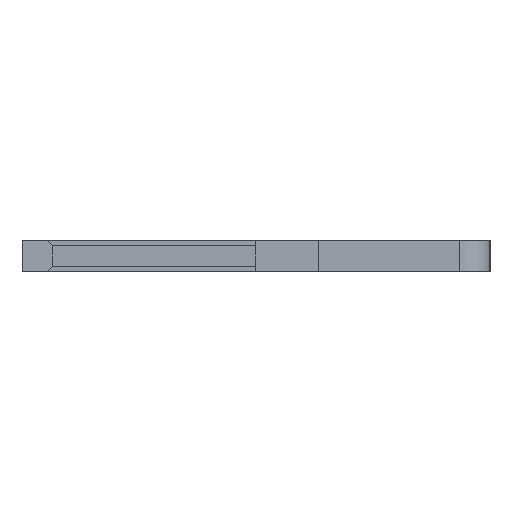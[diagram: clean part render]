
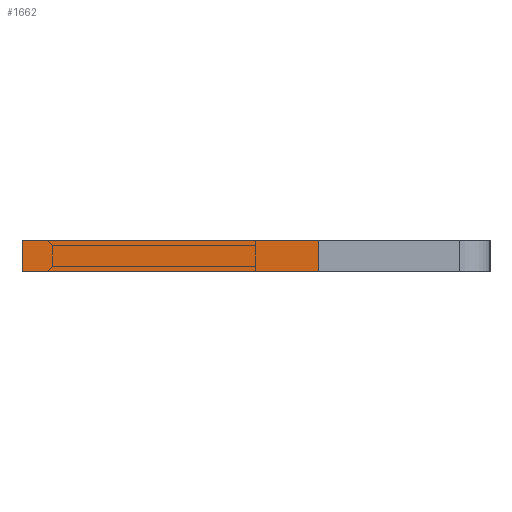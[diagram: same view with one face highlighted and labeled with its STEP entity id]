
A CAD part, left-side view. The second image highlights one B-rep face of the part: STEP entity #1662.
In plain terms, the highlighted face is planar.
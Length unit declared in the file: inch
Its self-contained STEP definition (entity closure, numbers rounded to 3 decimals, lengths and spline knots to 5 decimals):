
#30 = EDGE_CURVE ( 'NONE', #1767, #57, #1010, .T. ) ;
#57 = VERTEX_POINT ( 'NONE', #2047 ) ;
#97 = VECTOR ( 'NONE', #1008, 39.37008 ) ;
#149 = DIRECTION ( 'NONE',  ( 0., 0., 1. ) ) ;
#417 = DIRECTION ( 'NONE',  ( 0., 1., 0. ) ) ;
#457 = CARTESIAN_POINT ( 'NONE',  ( 0.01, 0.15, -0.04 ) ) ;
#492 = FACE_OUTER_BOUND ( 'NONE', #2109, .T. ) ;
#567 = LINE ( 'NONE', #1866, #97 ) ;
#683 = ORIENTED_EDGE ( 'NONE', *, *, #30, .F. ) ;
#798 = LINE ( 'NONE', #1511, #913 ) ;
#806 = EDGE_CURVE ( 'NONE', #2114, #57, #1166, .T. ) ;
#818 = DIRECTION ( 'NONE',  ( 1., 0., 0. ) ) ;
#913 = VECTOR ( 'NONE', #1022, 39.37008 ) ;
#996 = VERTEX_POINT ( 'NONE', #1268 ) ;
#1008 = DIRECTION ( 'NONE',  ( -1., 0., 0. ) ) ;
#1010 = LINE ( 'NONE', #1528, #1907 ) ;
#1022 = DIRECTION ( 'NONE',  ( 0., 1., 0. ) ) ;
#1028 = CARTESIAN_POINT ( 'NONE',  ( -0.01, -0.04, -0.04 ) ) ;
#1048 = AXIS2_PLACEMENT_3D ( 'NONE', #457, #149, #818 ) ;
#1166 = LINE ( 'NONE', #1278, #2105 ) ;
#1176 = ORIENTED_EDGE ( 'NONE', *, *, #1977, .F. ) ;
#1268 = CARTESIAN_POINT ( 'NONE',  ( 0.01, -0.04, -0.04 ) ) ;
#1278 = CARTESIAN_POINT ( 'NONE',  ( -0.01, 0.15, -0.04 ) ) ;
#1342 = PLANE ( 'NONE',  #1048 ) ;
#1493 = CARTESIAN_POINT ( 'NONE',  ( 0.01, 0.15, -0.04 ) ) ;
#1511 = CARTESIAN_POINT ( 'NONE',  ( 0.01, 0.15, -0.04 ) ) ;
#1528 = CARTESIAN_POINT ( 'NONE',  ( 0.01, 0.15, -0.04 ) ) ;
#1531 = ORIENTED_EDGE ( 'NONE', *, *, #1799, .T. ) ;
#1547 = DIRECTION ( 'NONE',  ( -1., 0., 0. ) ) ;
#1662 = ADVANCED_FACE ( 'NONE', ( #492 ), #1342, .F. ) ;
#1767 = VERTEX_POINT ( 'NONE', #1493 ) ;
#1799 = EDGE_CURVE ( 'NONE', #996, #2114, #567, .T. ) ;
#1805 = ORIENTED_EDGE ( 'NONE', *, *, #806, .T. ) ;
#1866 = CARTESIAN_POINT ( 'NONE',  ( 0.01, -0.04, -0.04 ) ) ;
#1907 = VECTOR ( 'NONE', #1547, 39.37008 ) ;
#1977 = EDGE_CURVE ( 'NONE', #996, #1767, #798, .T. ) ;
#2047 = CARTESIAN_POINT ( 'NONE',  ( -0.01, 0.15, -0.04 ) ) ;
#2105 = VECTOR ( 'NONE', #417, 39.37008 ) ;
#2109 = EDGE_LOOP ( 'NONE', ( #1805, #683, #1176, #1531 ) ) ;
#2114 = VERTEX_POINT ( 'NONE', #1028 ) ;
